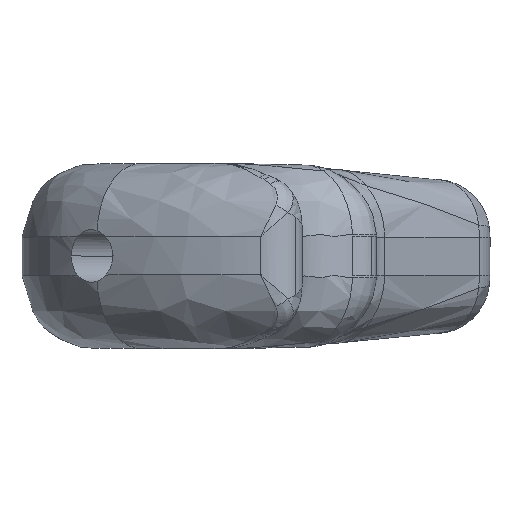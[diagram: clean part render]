
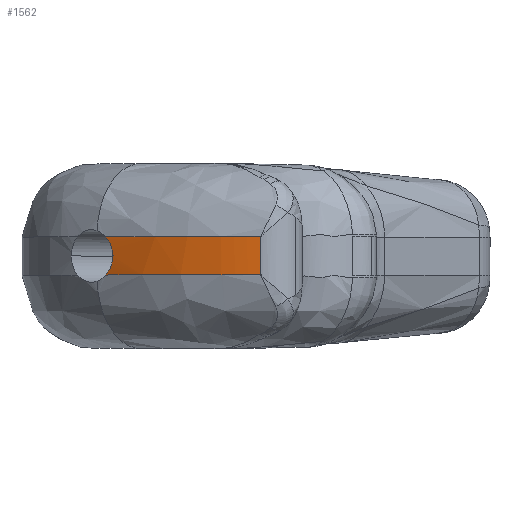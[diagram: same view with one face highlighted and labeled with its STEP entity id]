
A CAD part, top view. The second image highlights one B-rep face of the part: STEP entity #1562.
In plain terms, the highlighted cylindrical face has radius 63.5 mm (diameter 127 mm), a partial arc.
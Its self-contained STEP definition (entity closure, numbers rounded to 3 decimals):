
#136 = B_SPLINE_CURVE_WITH_KNOTS ( 'NONE', 3,
 ( #3249, #7384, #4528, #761, #5178 ),
 .UNSPECIFIED., .F., .F.,
 ( 4, 1, 4 ),
 ( 0., 0.814, 1. ),
 .UNSPECIFIED. ) ;
#172 = DIRECTION ( 'NONE',  ( 0., 1., 0. ) ) ;
#178 = CARTESIAN_POINT ( 'NONE',  ( -93.678, 11.857, 43.913 ) ) ;
#202 = CARTESIAN_POINT ( 'NONE',  ( -57.845, -7.234, -8.511 ) ) ;
#206 = CARTESIAN_POINT ( 'NONE',  ( -93.864, 5.466, 43.785 ) ) ;
#290 = ORIENTED_EDGE ( 'NONE', *, *, #8105, .F. ) ;
#522 = CARTESIAN_POINT ( 'NONE',  ( -73.997, 5.466, 52.9 ) ) ;
#672 = EDGE_CURVE ( 'NONE', #6853, #7358, #2382, .T. ) ;
#734 = DIRECTION ( 'NONE',  ( 0., 1., 0. ) ) ;
#761 = CARTESIAN_POINT ( 'NONE',  ( -74.74, 12.07, 52.705 ) ) ;
#825 = CARTESIAN_POINT ( 'NONE',  ( -93.513, 5.913, 44.026 ) ) ;
#873 = CARTESIAN_POINT ( 'NONE',  ( -93.864, 5.466, 43.785 ) ) ;
#894 = B_SPLINE_CURVE_WITH_KNOTS ( 'NONE', 3,
 ( #206, #3955, #825, #5244, #1441, #5870, #2078, #6488, #2710, #7133 ),
 .UNSPECIFIED., .F., .F.,
 ( 4, 2, 2, 2, 4 ),
 ( 0., 0.001, 0.002, 0.003, 0.004 ),
 .UNSPECIFIED. ) ;
#963 = B_SPLINE_CURVE_WITH_KNOTS ( 'NONE', 3,
 ( #6587, #2807, #5998, #2221, #6629 ),
 .UNSPECIFIED., .F., .F.,
 ( 4, 1, 4 ),
 ( 0.169, 0.896, 1. ),
 .UNSPECIFIED. ) ;
#1007 = B_SPLINE_CURVE_WITH_KNOTS ( 'NONE', 3,
 ( #7685, #3263, #6440, #2658, #7079, #3288, #7712, #3931, #178, #4571 ),
 .UNSPECIFIED., .F., .F.,
 ( 4, 2, 2, 2, 4 ),
 ( 0.004, 0.005, 0.006, 0.006, 0.007 ),
 .UNSPECIFIED. ) ;
#1247 = CARTESIAN_POINT ( 'NONE',  ( -57.845, 12.07, -8.511 ) ) ;
#1257 = CARTESIAN_POINT ( 'NONE',  ( -93.864, 5.466, 43.785 ) ) ;
#1344 = CARTESIAN_POINT ( 'NONE',  ( -67.132, -7.234, 54.306 ) ) ;
#1441 = CARTESIAN_POINT ( 'NONE',  ( -93.094, 6.688, 44.307 ) ) ;
#1490 = CARTESIAN_POINT ( 'NONE',  ( -87.654, 5.466, 47.677 ) ) ;
#1562 = ADVANCED_FACE ( 'NONE', ( #4859 ), #8008, .T. ) ;
#1877 = DIRECTION ( 'NONE',  ( 0.574, 0., -0.819 ) ) ;
#1905 = B_SPLINE_CURVE_WITH_KNOTS ( 'NONE', 3,
 ( #522, #4292, #2404, #6812 ),
 .UNSPECIFIED., .F., .F.,
 ( 4, 4 ),
 ( 0.247, 0.25 ),
 .UNSPECIFIED. ) ;
#2078 = CARTESIAN_POINT ( 'NONE',  ( -92.814, 7.547, 44.493 ) ) ;
#2197 = VERTEX_POINT ( 'NONE', #2331 ) ;
#2200 = EDGE_CURVE ( 'NONE', #4283, #6342, #136, .T. ) ;
#2221 = CARTESIAN_POINT ( 'NONE',  ( -85.749, 12.07, 48.531 ) ) ;
#2331 = CARTESIAN_POINT ( 'NONE',  ( -93.864, 12.07, 43.785 ) ) ;
#2370 = EDGE_CURVE ( 'NONE', #3264, #2197, #1007, .T. ) ;
#2382 = B_SPLINE_CURVE_WITH_KNOTS ( 'NONE', 3,
 ( #873, #5919, #1490, #6536, #2758, #7178 ),
 .UNSPECIFIED., .F., .F.,
 ( 4, 2, 4 ),
 ( 0.081, 0.54, 1. ),
 .UNSPECIFIED. ) ;
#2404 = CARTESIAN_POINT ( 'NONE',  ( -73.769, 5.466, 52.96 ) ) ;
#2555 = VERTEX_POINT ( 'NONE', #3570 ) ;
#2658 = CARTESIAN_POINT ( 'NONE',  ( -92.814, 9.989, 44.493 ) ) ;
#2710 = CARTESIAN_POINT ( 'NONE',  ( -92.684, 8.461, 44.579 ) ) ;
#2758 = CARTESIAN_POINT ( 'NONE',  ( -77.538, 5.466, 51.969 ) ) ;
#2795 = DIRECTION ( 'NONE',  ( 0., -1., 0. ) ) ;
#2807 = CARTESIAN_POINT ( 'NONE',  ( -91.57, 12.07, 45.365 ) ) ;
#2986 = VECTOR ( 'NONE', #734, 1000. ) ;
#3249 = CARTESIAN_POINT ( 'NONE',  ( -85.369, 12.07, 48.714 ) ) ;
#3263 = CARTESIAN_POINT ( 'NONE',  ( -92.684, 9.075, 44.579 ) ) ;
#3264 = VERTEX_POINT ( 'NONE', #3640 ) ;
#3288 = CARTESIAN_POINT ( 'NONE',  ( -93.093, 10.845, 44.308 ) ) ;
#3311 = EDGE_CURVE ( 'NONE', #7358, #2555, #1905, .T. ) ;
#3409 = ORIENTED_EDGE ( 'NONE', *, *, #4230, .F. ) ;
#3458 = CIRCLE ( 'NONE', #7859, 63.5 ) ;
#3570 = CARTESIAN_POINT ( 'NONE',  ( -73.655, 5.466, 52.989 ) ) ;
#3640 = CARTESIAN_POINT ( 'NONE',  ( -92.684, 8.768, 44.579 ) ) ;
#3712 = EDGE_CURVE ( 'NONE', #3901, #7994, #7610, .T. ) ;
#3898 = CARTESIAN_POINT ( 'NONE',  ( -85.369, 12.07, 48.714 ) ) ;
#3901 = VERTEX_POINT ( 'NONE', #4091 ) ;
#3931 = CARTESIAN_POINT ( 'NONE',  ( -93.512, 11.623, 44.026 ) ) ;
#3951 = DIRECTION ( 'NONE',  ( 0.819, 0., 0.574 ) ) ;
#3955 = CARTESIAN_POINT ( 'NONE',  ( -93.678, 5.68, 43.913 ) ) ;
#3966 = EDGE_LOOP ( 'NONE', ( #290, #5670, #6359, #5735, #4778, #3409, #4289, #6113, #6596 ) ) ;
#4040 = EDGE_CURVE ( 'NONE', #2197, #4283, #963, .T. ) ;
#4091 = CARTESIAN_POINT ( 'NONE',  ( -67.132, 5.466, 54.306 ) ) ;
#4230 = EDGE_CURVE ( 'NONE', #6342, #7994, #3458, .T. ) ;
#4283 = VERTEX_POINT ( 'NONE', #3898 ) ;
#4288 = AXIS2_PLACEMENT_3D ( 'NONE', #202, #172, #3951 ) ;
#4289 = ORIENTED_EDGE ( 'NONE', *, *, #2200, .F. ) ;
#4292 = CARTESIAN_POINT ( 'NONE',  ( -73.883, 5.466, 52.93 ) ) ;
#4528 = CARTESIAN_POINT ( 'NONE',  ( -78.711, 12.07, 51.582 ) ) ;
#4571 = CARTESIAN_POINT ( 'NONE',  ( -93.864, 12.07, 43.785 ) ) ;
#4741 = AXIS2_PLACEMENT_3D ( 'NONE', #6573, #2795, #7225 ) ;
#4770 = CARTESIAN_POINT ( 'NONE',  ( -73.997, 5.466, 52.9 ) ) ;
#4778 = ORIENTED_EDGE ( 'NONE', *, *, #3712, .T. ) ;
#4859 = FACE_OUTER_BOUND ( 'NONE', #3966, .T. ) ;
#5103 = EDGE_CURVE ( 'NONE', #3901, #2555, #6917, .T. ) ;
#5178 = CARTESIAN_POINT ( 'NONE',  ( -73.997, 12.07, 52.9 ) ) ;
#5244 = CARTESIAN_POINT ( 'NONE',  ( -93.221, 6.415, 44.223 ) ) ;
#5460 = CARTESIAN_POINT ( 'NONE',  ( -73.997, 12.07, 52.9 ) ) ;
#5670 = ORIENTED_EDGE ( 'NONE', *, *, #672, .T. ) ;
#5675 = DIRECTION ( 'NONE',  ( 0., 1., 0. ) ) ;
#5735 = ORIENTED_EDGE ( 'NONE', *, *, #5103, .F. ) ;
#5870 = CARTESIAN_POINT ( 'NONE',  ( -92.891, 7.254, 44.442 ) ) ;
#5919 = CARTESIAN_POINT ( 'NONE',  ( -90.849, 5.466, 45.862 ) ) ;
#5998 = CARTESIAN_POINT ( 'NONE',  ( -88.758, 12.07, 47.047 ) ) ;
#6113 = ORIENTED_EDGE ( 'NONE', *, *, #4040, .F. ) ;
#6342 = VERTEX_POINT ( 'NONE', #5460 ) ;
#6359 = ORIENTED_EDGE ( 'NONE', *, *, #3311, .T. ) ;
#6440 = CARTESIAN_POINT ( 'NONE',  ( -92.709, 9.381, 44.562 ) ) ;
#6488 = CARTESIAN_POINT ( 'NONE',  ( -92.71, 8.15, 44.562 ) ) ;
#6536 = CARTESIAN_POINT ( 'NONE',  ( -80.998, 5.466, 50.731 ) ) ;
#6573 = CARTESIAN_POINT ( 'NONE',  ( -57.845, 5.466, -8.511 ) ) ;
#6587 = CARTESIAN_POINT ( 'NONE',  ( -93.864, 12.07, 43.785 ) ) ;
#6596 = ORIENTED_EDGE ( 'NONE', *, *, #2370, .F. ) ;
#6629 = CARTESIAN_POINT ( 'NONE',  ( -85.369, 12.07, 48.714 ) ) ;
#6812 = CARTESIAN_POINT ( 'NONE',  ( -73.655, 5.466, 52.989 ) ) ;
#6853 = VERTEX_POINT ( 'NONE', #1257 ) ;
#6900 = CARTESIAN_POINT ( 'NONE',  ( -67.132, 12.07, 54.306 ) ) ;
#6917 = CIRCLE ( 'NONE', #4741, 63.5 ) ;
#7079 = CARTESIAN_POINT ( 'NONE',  ( -92.891, 10.282, 44.442 ) ) ;
#7133 = CARTESIAN_POINT ( 'NONE',  ( -92.684, 8.768, 44.579 ) ) ;
#7178 = CARTESIAN_POINT ( 'NONE',  ( -73.997, 5.466, 52.9 ) ) ;
#7225 = DIRECTION ( 'NONE',  ( -0.574, 0., 0.819 ) ) ;
#7358 = VERTEX_POINT ( 'NONE', #4770 ) ;
#7384 = CARTESIAN_POINT ( 'NONE',  ( -82.478, 12.07, 50.104 ) ) ;
#7610 = LINE ( 'NONE', #1344, #2986 ) ;
#7685 = CARTESIAN_POINT ( 'NONE',  ( -92.684, 8.768, 44.579 ) ) ;
#7712 = CARTESIAN_POINT ( 'NONE',  ( -93.219, 11.118, 44.224 ) ) ;
#7859 = AXIS2_PLACEMENT_3D ( 'NONE', #1247, #5675, #1877 ) ;
#7994 = VERTEX_POINT ( 'NONE', #6900 ) ;
#8008 = CYLINDRICAL_SURFACE ( 'NONE', #4288, 63.5 ) ;
#8105 = EDGE_CURVE ( 'NONE', #6853, #3264, #894, .T. ) ;
